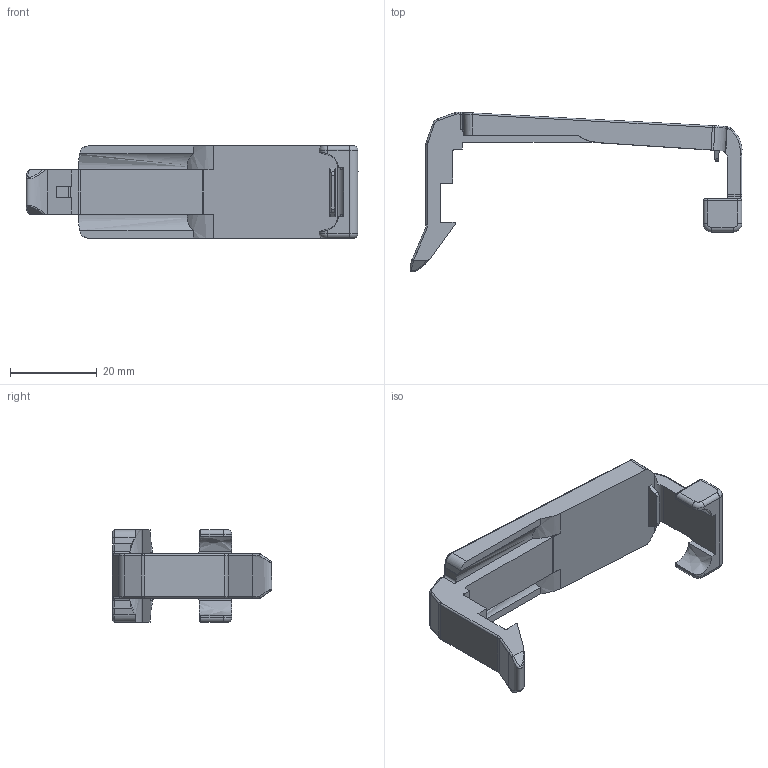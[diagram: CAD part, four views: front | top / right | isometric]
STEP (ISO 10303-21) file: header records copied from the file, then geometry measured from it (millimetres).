
FILE_DESCRIPTION (( 'STEP AP214' ), '1' );
FILE_NAME ('Dust_Cover.STEP', '2022-09-24T15:53:39', ( '' ), ( '' ), 'SwSTEP 2.0', 'SolidWorks 2021', '' );
FILE_SCHEMA (( 'AUTOMOTIVE_DESIGN' ));
Length unit declared in the file: millimetre
Products named in the file (1): Dust_Cover
Bounding box: 76.69 x 36.85 x 21.3 mm (x, y, z)
Volume: 9902.7 mm3; surface area: 5730.6 mm2
Topology: 1 solids, 1 shells, 175 faces, 453 edges, 281 vertices
Faces by surface type: cylinder 66, plane 57, torus 26, bspline 26
Entity records: 6179 total; most frequent: CARTESIAN_POINT 2068, ORIENTED_EDGE 906, DIRECTION 798, EDGE_CURVE 453, AXIS2_PLACEMENT_3D 285, VERTEX_POINT 281, VECTOR 228, LINE 228
